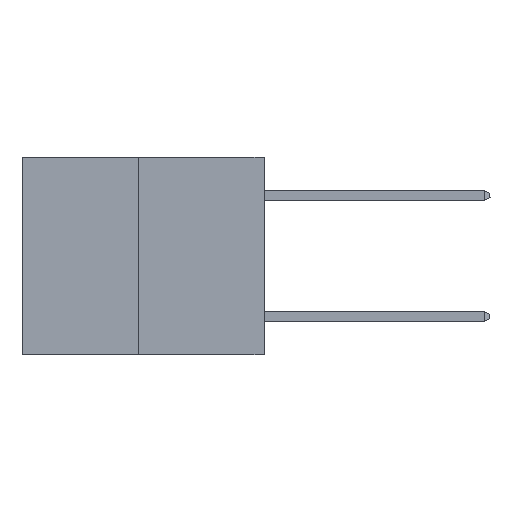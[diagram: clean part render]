
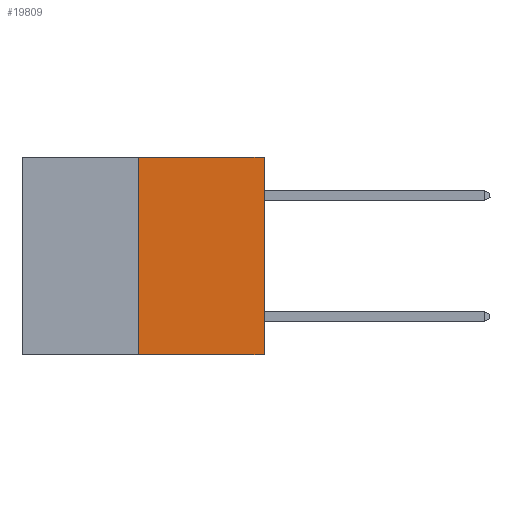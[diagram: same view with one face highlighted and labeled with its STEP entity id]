
A CAD part, left-side view. The second image highlights one B-rep face of the part: STEP entity #19809.
In plain terms, the highlighted planar face has unit normal (-1, 0, 0).
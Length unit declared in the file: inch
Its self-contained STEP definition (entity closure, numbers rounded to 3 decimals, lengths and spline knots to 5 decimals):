
#2554 = VERTEX_POINT ( 'NONE', #5530 ) ;
#2834 = VECTOR ( 'NONE', #4650, 39.37008 ) ;
#2977 = PLANE ( 'NONE',  #10298 ) ;
#3613 = EDGE_CURVE ( 'NONE', #22190, #8462, #18142, .T. ) ;
#4650 = DIRECTION ( 'NONE',  ( 0., 0., 1. ) ) ;
#4840 = CARTESIAN_POINT ( 'NONE',  ( 0., 0., 0. ) ) ;
#5454 = LINE ( 'NONE', #22286, #9484 ) ;
#5530 = CARTESIAN_POINT ( 'NONE',  ( 0., 0.312, -0.49 ) ) ;
#6048 = DIRECTION ( 'NONE',  ( 0., -1., 0. ) ) ;
#6974 = ORIENTED_EDGE ( 'NONE', *, *, #3613, .T. ) ;
#7107 = VECTOR ( 'NONE', #13580, 39.37008 ) ;
#7874 = CARTESIAN_POINT ( 'NONE',  ( 0., 0., -0.49 ) ) ;
#8462 = VERTEX_POINT ( 'NONE', #25787 ) ;
#9333 = CARTESIAN_POINT ( 'NONE',  ( 0., 0.6, -0.49 ) ) ;
#9484 = VECTOR ( 'NONE', #6048, 39.37008 ) ;
#10171 = EDGE_CURVE ( 'NONE', #2554, #10588, #22767, .T. ) ;
#10298 = AXIS2_PLACEMENT_3D ( 'NONE', #26748, #12311, #21719 ) ;
#10588 = VERTEX_POINT ( 'NONE', #23853 ) ;
#10826 = ORIENTED_EDGE ( 'NONE', *, *, #20888, .F. ) ;
#11278 = EDGE_LOOP ( 'NONE', ( #24558, #27607, #6974, #10826 ) ) ;
#12311 = DIRECTION ( 'NONE',  ( 1., 0., 0. ) ) ;
#13580 = DIRECTION ( 'NONE',  ( 0., -1., 0. ) ) ;
#15050 = VECTOR ( 'NONE', #28444, 39.37008 ) ;
#18142 = LINE ( 'NONE', #4840, #2834 ) ;
#19809 = ADVANCED_FACE ( 'NONE', ( #26006 ), #2977, .F. ) ;
#20888 = EDGE_CURVE ( 'NONE', #10588, #8462, #5454, .T. ) ;
#20950 = LINE ( 'NONE', #9333, #7107 ) ;
#21719 = DIRECTION ( 'NONE',  ( 0., 0., -1. ) ) ;
#22190 = VERTEX_POINT ( 'NONE', #7874 ) ;
#22286 = CARTESIAN_POINT ( 'NONE',  ( 0., 0.6, 0. ) ) ;
#22767 = LINE ( 'NONE', #28249, #15050 ) ;
#23853 = CARTESIAN_POINT ( 'NONE',  ( 0., 0.312, 0. ) ) ;
#24558 = ORIENTED_EDGE ( 'NONE', *, *, #10171, .F. ) ;
#24747 = EDGE_CURVE ( 'NONE', #2554, #22190, #20950, .T. ) ;
#25787 = CARTESIAN_POINT ( 'NONE',  ( 0., 0., 0. ) ) ;
#26006 = FACE_OUTER_BOUND ( 'NONE', #11278, .T. ) ;
#26748 = CARTESIAN_POINT ( 'NONE',  ( 0., 0.6, 0. ) ) ;
#27607 = ORIENTED_EDGE ( 'NONE', *, *, #24747, .T. ) ;
#28249 = CARTESIAN_POINT ( 'NONE',  ( 0., 0.312, -0.49 ) ) ;
#28444 = DIRECTION ( 'NONE',  ( 0., 0., 1. ) ) ;
